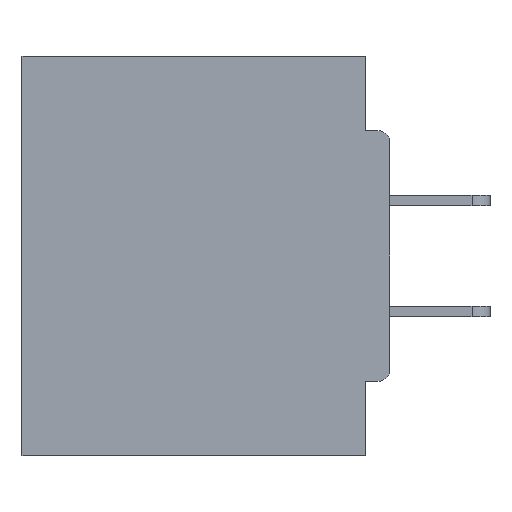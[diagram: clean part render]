
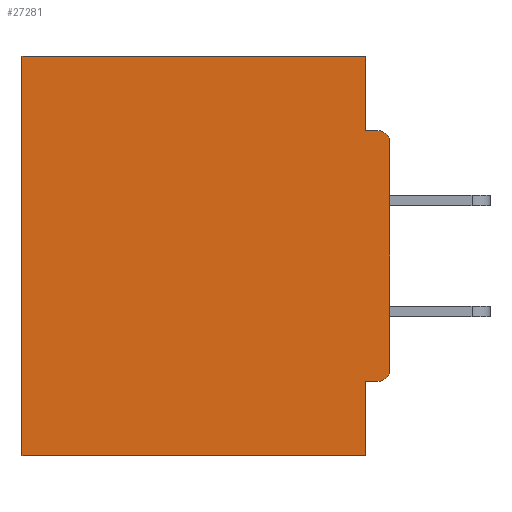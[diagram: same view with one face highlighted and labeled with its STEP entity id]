
A CAD part, left-side view. The second image highlights one B-rep face of the part: STEP entity #27281.
In plain terms, the highlighted planar face has unit normal (-1, 0, 0).
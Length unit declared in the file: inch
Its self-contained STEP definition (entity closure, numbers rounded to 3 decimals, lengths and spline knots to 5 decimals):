
#43 = DIRECTION ( 'NONE',  ( 0., 0., -1. ) ) ;
#107 = CARTESIAN_POINT ( 'NONE',  ( 0.298, 0., 0. ) ) ;
#386 = VECTOR ( 'NONE', #14640, 39.37008 ) ;
#812 = LINE ( 'NONE', #33534, #386 ) ;
#1223 = VERTEX_POINT ( 'NONE', #30638 ) ;
#1499 = VECTOR ( 'NONE', #28477, 39.37008 ) ;
#4027 = EDGE_CURVE ( 'NONE', #19434, #23901, #33628, .T. ) ;
#4335 = CIRCLE ( 'NONE', #24688, 0.015 ) ;
#5263 = CARTESIAN_POINT ( 'NONE',  ( 0.298, 0.46, -0.5 ) ) ;
#6796 = EDGE_CURVE ( 'NONE', #24495, #1223, #812, .T. ) ;
#7678 = ORIENTED_EDGE ( 'NONE', *, *, #28050, .F. ) ;
#7733 = CARTESIAN_POINT ( 'NONE',  ( 0.298, 0.031, -0.5 ) ) ;
#7972 = CARTESIAN_POINT ( 'NONE',  ( 0.298, 0.031, 0. ) ) ;
#8077 = PLANE ( 'NONE',  #35335 ) ;
#9307 = CARTESIAN_POINT ( 'NONE',  ( 0.298, 0.015, -0.0935 ) ) ;
#9452 = CIRCLE ( 'NONE', #18223, 0.015 ) ;
#9904 = VECTOR ( 'NONE', #26749, 39.37008 ) ;
#10549 = VERTEX_POINT ( 'NONE', #20004 ) ;
#10708 = LINE ( 'NONE', #24651, #30845 ) ;
#10867 = VERTEX_POINT ( 'NONE', #35477 ) ;
#11342 = VECTOR ( 'NONE', #25702, 39.37008 ) ;
#11678 = VECTOR ( 'NONE', #30055, 39.37008 ) ;
#12121 = LINE ( 'NONE', #107, #11678 ) ;
#12254 = FACE_OUTER_BOUND ( 'NONE', #24757, .T. ) ;
#12974 = VECTOR ( 'NONE', #21494, 39.37008 ) ;
#13330 = VERTEX_POINT ( 'NONE', #26357 ) ;
#13474 = LINE ( 'NONE', #33852, #11342 ) ;
#14640 = DIRECTION ( 'NONE',  ( 0., 1., 0. ) ) ;
#15334 = ORIENTED_EDGE ( 'NONE', *, *, #23700, .T. ) ;
#15436 = CARTESIAN_POINT ( 'NONE',  ( 0.298, 0., -0.1085 ) ) ;
#15689 = CARTESIAN_POINT ( 'NONE',  ( 0.298, 0., -0.0935 ) ) ;
#15708 = VECTOR ( 'NONE', #29109, 39.37008 ) ;
#15728 = EDGE_CURVE ( 'NONE', #31876, #10867, #20200, .T. ) ;
#15738 = ORIENTED_EDGE ( 'NONE', *, *, #19840, .T. ) ;
#16342 = CARTESIAN_POINT ( 'NONE',  ( 0.298, 0., 0. ) ) ;
#17431 = CARTESIAN_POINT ( 'NONE',  ( 0.298, 0.015, -0.4065 ) ) ;
#17640 = VERTEX_POINT ( 'NONE', #7972 ) ;
#18222 = DIRECTION ( 'NONE',  ( 0., 0., -1. ) ) ;
#18223 = AXIS2_PLACEMENT_3D ( 'NONE', #26707, #18346, #18222 ) ;
#18346 = DIRECTION ( 'NONE',  ( -1., 0., 0. ) ) ;
#19434 = VERTEX_POINT ( 'NONE', #21604 ) ;
#19782 = EDGE_CURVE ( 'NONE', #24495, #10867, #9452, .T. ) ;
#19840 = EDGE_CURVE ( 'NONE', #13330, #23901, #10708, .T. ) ;
#20004 = CARTESIAN_POINT ( 'NONE',  ( 0.298, 0.031, -0.0935 ) ) ;
#20200 = LINE ( 'NONE', #35125, #9904 ) ;
#20712 = ORIENTED_EDGE ( 'NONE', *, *, #34953, .T. ) ;
#21188 = ORIENTED_EDGE ( 'NONE', *, *, #21585, .F. ) ;
#21486 = DIRECTION ( 'NONE',  ( 1., 0., 0. ) ) ;
#21494 = DIRECTION ( 'NONE',  ( 0., 0., -1. ) ) ;
#21585 = EDGE_CURVE ( 'NONE', #10549, #28059, #23852, .T. ) ;
#21604 = CARTESIAN_POINT ( 'NONE',  ( 0.298, 0.031, -0.5 ) ) ;
#23700 = EDGE_CURVE ( 'NONE', #17640, #13330, #12121, .T. ) ;
#23852 = LINE ( 'NONE', #15689, #15708 ) ;
#23901 = VERTEX_POINT ( 'NONE', #5263 ) ;
#23939 = ORIENTED_EDGE ( 'NONE', *, *, #6796, .F. ) ;
#24495 = VERTEX_POINT ( 'NONE', #17431 ) ;
#24538 = ORIENTED_EDGE ( 'NONE', *, *, #15728, .F. ) ;
#24651 = CARTESIAN_POINT ( 'NONE',  ( 0.298, 0.46, 0. ) ) ;
#24688 = AXIS2_PLACEMENT_3D ( 'NONE', #30835, #30712, #25314 ) ;
#24757 = EDGE_LOOP ( 'NONE', ( #20712, #21188, #7678, #15334, #15738, #33271, #26448, #23939, #32029, #24538 ) ) ;
#25314 = DIRECTION ( 'NONE',  ( 0., 0., -1. ) ) ;
#25702 = DIRECTION ( 'NONE',  ( 0., 0., -1. ) ) ;
#26357 = CARTESIAN_POINT ( 'NONE',  ( 0.298, 0.46, 0. ) ) ;
#26448 = ORIENTED_EDGE ( 'NONE', *, *, #34712, .F. ) ;
#26707 = CARTESIAN_POINT ( 'NONE',  ( 0.298, 0.015, -0.3915 ) ) ;
#26749 = DIRECTION ( 'NONE',  ( 0., 0., -1. ) ) ;
#27281 = ADVANCED_FACE ( 'NONE', ( #12254 ), #8077, .F. ) ;
#27526 = DIRECTION ( 'NONE',  ( 0., 0., -1. ) ) ;
#28050 = EDGE_CURVE ( 'NONE', #17640, #10549, #13474, .T. ) ;
#28059 = VERTEX_POINT ( 'NONE', #9307 ) ;
#28477 = DIRECTION ( 'NONE',  ( 0., 1., 0. ) ) ;
#28599 = CARTESIAN_POINT ( 'NONE',  ( 0.298, 0., -0.5 ) ) ;
#29109 = DIRECTION ( 'NONE',  ( 0., -1., 0. ) ) ;
#30055 = DIRECTION ( 'NONE',  ( 0., 1., 0. ) ) ;
#30638 = CARTESIAN_POINT ( 'NONE',  ( 0.298, 0.031, -0.4065 ) ) ;
#30712 = DIRECTION ( 'NONE',  ( -1., 0., 0. ) ) ;
#30835 = CARTESIAN_POINT ( 'NONE',  ( 0.298, 0.015, -0.1085 ) ) ;
#30845 = VECTOR ( 'NONE', #27526, 39.37008 ) ;
#31420 = LINE ( 'NONE', #7733, #12974 ) ;
#31876 = VERTEX_POINT ( 'NONE', #15436 ) ;
#32029 = ORIENTED_EDGE ( 'NONE', *, *, #19782, .T. ) ;
#33271 = ORIENTED_EDGE ( 'NONE', *, *, #4027, .F. ) ;
#33534 = CARTESIAN_POINT ( 'NONE',  ( 0.298, 0., -0.4065 ) ) ;
#33628 = LINE ( 'NONE', #28599, #1499 ) ;
#33852 = CARTESIAN_POINT ( 'NONE',  ( 0.298, 0.031, -0.5 ) ) ;
#34712 = EDGE_CURVE ( 'NONE', #1223, #19434, #31420, .T. ) ;
#34953 = EDGE_CURVE ( 'NONE', #31876, #28059, #4335, .T. ) ;
#35125 = CARTESIAN_POINT ( 'NONE',  ( 0.298, 0., 0. ) ) ;
#35335 = AXIS2_PLACEMENT_3D ( 'NONE', #16342, #21486, #43 ) ;
#35477 = CARTESIAN_POINT ( 'NONE',  ( 0.298, 0., -0.3915 ) ) ;
